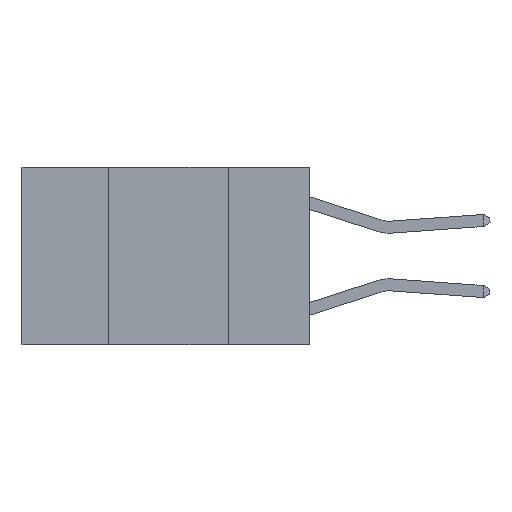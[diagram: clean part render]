
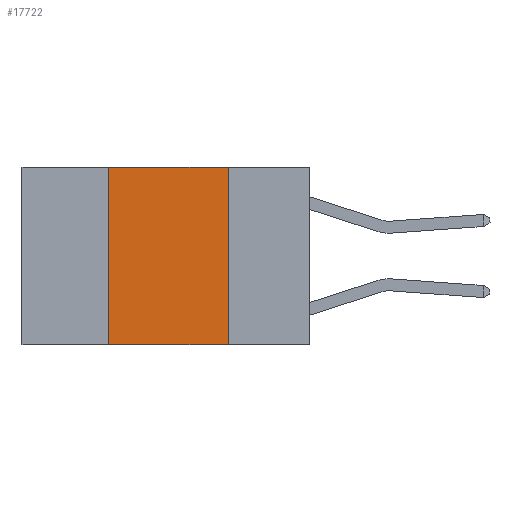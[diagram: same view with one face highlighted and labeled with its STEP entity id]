
A CAD part, left-side view. The second image highlights one B-rep face of the part: STEP entity #17722.
In plain terms, the highlighted planar face has unit normal (-1, 0, 0).
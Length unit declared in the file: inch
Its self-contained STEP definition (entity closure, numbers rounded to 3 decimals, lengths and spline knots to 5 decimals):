
#191 = LINE ( 'NONE', #23076, #5486 ) ;
#3423 = ORIENTED_EDGE ( 'NONE', *, *, #14459, .T. ) ;
#4214 = ORIENTED_EDGE ( 'NONE', *, *, #20277, .F. ) ;
#4552 = LINE ( 'NONE', #14892, #19795 ) ;
#4979 = DIRECTION ( 'NONE',  ( 0., 0., -1. ) ) ;
#5476 = CARTESIAN_POINT ( 'NONE',  ( 0., 0.6, 0. ) ) ;
#5486 = VECTOR ( 'NONE', #11198, 39.37008 ) ;
#6642 = EDGE_CURVE ( 'NONE', #11139, #7812, #10564, .T. ) ;
#7484 = DIRECTION ( 'NONE',  ( 1., 0., 0. ) ) ;
#7718 = CARTESIAN_POINT ( 'NONE',  ( 0., 0.6, 0. ) ) ;
#7812 = VERTEX_POINT ( 'NONE', #19409 ) ;
#8310 = ORIENTED_EDGE ( 'NONE', *, *, #6642, .F. ) ;
#9065 = EDGE_LOOP ( 'NONE', ( #4214, #10812, #8310, #3423 ) ) ;
#9726 = DIRECTION ( 'NONE',  ( 0., -1., 0. ) ) ;
#10072 = LINE ( 'NONE', #7718, #25270 ) ;
#10564 = LINE ( 'NONE', #18246, #14585 ) ;
#10812 = ORIENTED_EDGE ( 'NONE', *, *, #16383, .F. ) ;
#11139 = VERTEX_POINT ( 'NONE', #16350 ) ;
#11198 = DIRECTION ( 'NONE',  ( 0., -1., 0. ) ) ;
#14459 = EDGE_CURVE ( 'NONE', #11139, #23831, #191, .T. ) ;
#14585 = VECTOR ( 'NONE', #20241, 39.37008 ) ;
#14892 = CARTESIAN_POINT ( 'NONE',  ( 0., 0.17, 0. ) ) ;
#15578 = FACE_OUTER_BOUND ( 'NONE', #9065, .T. ) ;
#16350 = CARTESIAN_POINT ( 'NONE',  ( 0., 0.42, -0.37 ) ) ;
#16383 = EDGE_CURVE ( 'NONE', #7812, #25403, #10072, .T. ) ;
#17404 = PLANE ( 'NONE',  #25288 ) ;
#17476 = CARTESIAN_POINT ( 'NONE',  ( 0., 0.17, 0. ) ) ;
#17601 = CARTESIAN_POINT ( 'NONE',  ( 0., 0.17, -0.37 ) ) ;
#17722 = ADVANCED_FACE ( 'NONE', ( #15578 ), #17404, .F. ) ;
#18246 = CARTESIAN_POINT ( 'NONE',  ( 0., 0.42, 0. ) ) ;
#19409 = CARTESIAN_POINT ( 'NONE',  ( 0., 0.42, 0. ) ) ;
#19795 = VECTOR ( 'NONE', #4979, 39.37008 ) ;
#20241 = DIRECTION ( 'NONE',  ( 0., 0., 1. ) ) ;
#20277 = EDGE_CURVE ( 'NONE', #25403, #23831, #4552, .T. ) ;
#21388 = DIRECTION ( 'NONE',  ( 0., 0., -1. ) ) ;
#23076 = CARTESIAN_POINT ( 'NONE',  ( 0., 0.6, -0.37 ) ) ;
#23831 = VERTEX_POINT ( 'NONE', #17601 ) ;
#25270 = VECTOR ( 'NONE', #9726, 39.37008 ) ;
#25288 = AXIS2_PLACEMENT_3D ( 'NONE', #5476, #7484, #21388 ) ;
#25403 = VERTEX_POINT ( 'NONE', #17476 ) ;
